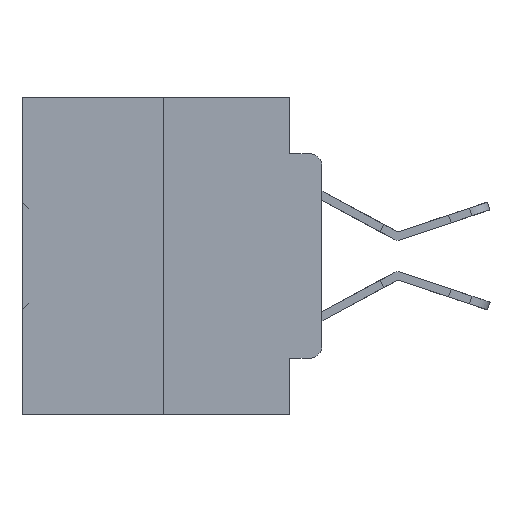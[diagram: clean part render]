
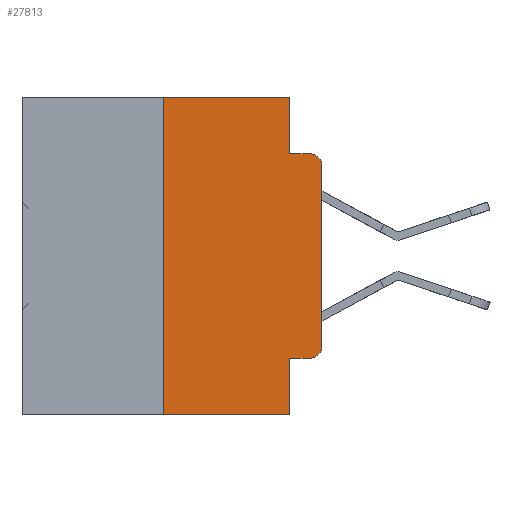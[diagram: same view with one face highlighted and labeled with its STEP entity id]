
A CAD part, left-side view. The second image highlights one B-rep face of the part: STEP entity #27813.
In plain terms, the highlighted planar face has unit normal (-1, 0, 0).
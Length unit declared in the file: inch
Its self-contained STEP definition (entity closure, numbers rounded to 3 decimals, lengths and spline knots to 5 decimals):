
#377 = CARTESIAN_POINT ( 'NONE',  ( 0., 0.02, -0.1085 ) ) ;
#458 = ORIENTED_EDGE ( 'NONE', *, *, #30787, .F. ) ;
#922 = EDGE_CURVE ( 'NONE', #39121, #20707, #31817, .T. ) ;
#1059 = ORIENTED_EDGE ( 'NONE', *, *, #10953, .T. ) ;
#1646 = AXIS2_PLACEMENT_3D ( 'NONE', #377, #25397, #3237 ) ;
#1842 = ORIENTED_EDGE ( 'NONE', *, *, #34282, .T. ) ;
#2222 = CARTESIAN_POINT ( 'NONE',  ( 0., 0.051, -0.4115 ) ) ;
#3047 = DIRECTION ( 'NONE',  ( 0., 0., -1. ) ) ;
#3237 = DIRECTION ( 'NONE',  ( 0., 0., -1. ) ) ;
#3352 = LINE ( 'NONE', #37410, #21330 ) ;
#3998 = ORIENTED_EDGE ( 'NONE', *, *, #922, .F. ) ;
#4607 = CARTESIAN_POINT ( 'NONE',  ( 0., 0.051, 0. ) ) ;
#4896 = VERTEX_POINT ( 'NONE', #10199 ) ;
#5140 = EDGE_CURVE ( 'NONE', #37113, #7721, #8567, .T. ) ;
#5470 = FACE_OUTER_BOUND ( 'NONE', #26288, .T. ) ;
#5707 = ORIENTED_EDGE ( 'NONE', *, *, #20006, .T. ) ;
#6182 = CARTESIAN_POINT ( 'NONE',  ( 0., 0.25, 0. ) ) ;
#6184 = ORIENTED_EDGE ( 'NONE', *, *, #12628, .F. ) ;
#6876 = CARTESIAN_POINT ( 'NONE',  ( 0., 0.051, -0.0885 ) ) ;
#7721 = VERTEX_POINT ( 'NONE', #10464 ) ;
#8567 = LINE ( 'NONE', #32364, #11851 ) ;
#8729 = CIRCLE ( 'NONE', #1646, 0.02 ) ;
#9619 = VERTEX_POINT ( 'NONE', #39249 ) ;
#10199 = CARTESIAN_POINT ( 'NONE',  ( 0., 0., -0.3915 ) ) ;
#10464 = CARTESIAN_POINT ( 'NONE',  ( 0., 0.02, -0.0885 ) ) ;
#10778 = CIRCLE ( 'NONE', #11408, 0.02 ) ;
#10953 = EDGE_CURVE ( 'NONE', #39121, #31346, #32854, .T. ) ;
#11408 = AXIS2_PLACEMENT_3D ( 'NONE', #16907, #32036, #20530 ) ;
#11587 = DIRECTION ( 'NONE',  ( 0., -1., 0. ) ) ;
#11851 = VECTOR ( 'NONE', #11587, 39.37008 ) ;
#12628 = EDGE_CURVE ( 'NONE', #38795, #37113, #25783, .T. ) ;
#13248 = DIRECTION ( 'NONE',  ( 0., 0., 1. ) ) ;
#13887 = CARTESIAN_POINT ( 'NONE',  ( 0., 0.051, 0. ) ) ;
#14482 = EDGE_CURVE ( 'NONE', #37508, #20707, #3352, .T. ) ;
#15506 = CARTESIAN_POINT ( 'NONE',  ( 0., 0.25, 0. ) ) ;
#16087 = DIRECTION ( 'NONE',  ( 0., 0., -1. ) ) ;
#16580 = ORIENTED_EDGE ( 'NONE', *, *, #14482, .T. ) ;
#16879 = ORIENTED_EDGE ( 'NONE', *, *, #5140, .F. ) ;
#16907 = CARTESIAN_POINT ( 'NONE',  ( 0., 0.02, -0.3915 ) ) ;
#17319 = CARTESIAN_POINT ( 'NONE',  ( 0., 0.473, 0. ) ) ;
#17368 = ORIENTED_EDGE ( 'NONE', *, *, #39757, .T. ) ;
#18345 = PLANE ( 'NONE',  #19386 ) ;
#18455 = DIRECTION ( 'NONE',  ( 0., 0., 1. ) ) ;
#18849 = DIRECTION ( 'NONE',  ( 0., -1., 0. ) ) ;
#19386 = AXIS2_PLACEMENT_3D ( 'NONE', #36103, #30049, #3047 ) ;
#20006 = EDGE_CURVE ( 'NONE', #9619, #7721, #8729, .T. ) ;
#20530 = DIRECTION ( 'NONE',  ( 0., 0., -1. ) ) ;
#20707 = VERTEX_POINT ( 'NONE', #31081 ) ;
#20748 = CARTESIAN_POINT ( 'NONE',  ( 0., 0.25, -0.5 ) ) ;
#20751 = DIRECTION ( 'NONE',  ( 0., -1., 0. ) ) ;
#20870 = VECTOR ( 'NONE', #20751, 39.37008 ) ;
#21330 = VECTOR ( 'NONE', #18849, 39.37008 ) ;
#23921 = VERTEX_POINT ( 'NONE', #15506 ) ;
#24989 = VECTOR ( 'NONE', #13248, 39.37008 ) ;
#25122 = VECTOR ( 'NONE', #35687, 39.37008 ) ;
#25397 = DIRECTION ( 'NONE',  ( -1., 0., 0. ) ) ;
#25742 = CARTESIAN_POINT ( 'NONE',  ( 0., 0., 0. ) ) ;
#25783 = LINE ( 'NONE', #13887, #26413 ) ;
#26288 = EDGE_LOOP ( 'NONE', ( #17368, #5707, #16879, #6184, #458, #37160, #16580, #3998, #1059, #1842 ) ) ;
#26413 = VECTOR ( 'NONE', #35250, 39.37008 ) ;
#27813 = ADVANCED_FACE ( 'NONE', ( #5470 ), #18345, .F. ) ;
#27913 = VECTOR ( 'NONE', #18455, 39.37008 ) ;
#28613 = CARTESIAN_POINT ( 'NONE',  ( 0., 0.051, -0.4115 ) ) ;
#30049 = DIRECTION ( 'NONE',  ( 1., 0., 0. ) ) ;
#30787 = EDGE_CURVE ( 'NONE', #23921, #38795, #36282, .T. ) ;
#31081 = CARTESIAN_POINT ( 'NONE',  ( 0., 0.051, -0.5 ) ) ;
#31346 = VERTEX_POINT ( 'NONE', #32608 ) ;
#31533 = EDGE_CURVE ( 'NONE', #37508, #23921, #33796, .T. ) ;
#31817 = LINE ( 'NONE', #4607, #33098 ) ;
#31980 = LINE ( 'NONE', #25742, #24989 ) ;
#32036 = DIRECTION ( 'NONE',  ( -1., 0., 0. ) ) ;
#32364 = CARTESIAN_POINT ( 'NONE',  ( 0., 0.051, -0.0885 ) ) ;
#32608 = CARTESIAN_POINT ( 'NONE',  ( 0., 0.02, -0.4115 ) ) ;
#32854 = LINE ( 'NONE', #2222, #25122 ) ;
#33098 = VECTOR ( 'NONE', #16087, 39.37008 ) ;
#33796 = LINE ( 'NONE', #6182, #27913 ) ;
#34282 = EDGE_CURVE ( 'NONE', #31346, #4896, #10778, .T. ) ;
#35250 = DIRECTION ( 'NONE',  ( 0., 0., -1. ) ) ;
#35687 = DIRECTION ( 'NONE',  ( 0., -1., 0. ) ) ;
#36103 = CARTESIAN_POINT ( 'NONE',  ( 0., 0.473, 0. ) ) ;
#36282 = LINE ( 'NONE', #17319, #20870 ) ;
#37113 = VERTEX_POINT ( 'NONE', #6876 ) ;
#37160 = ORIENTED_EDGE ( 'NONE', *, *, #31533, .F. ) ;
#37410 = CARTESIAN_POINT ( 'NONE',  ( 0., 0.473, -0.5 ) ) ;
#37508 = VERTEX_POINT ( 'NONE', #20748 ) ;
#38514 = CARTESIAN_POINT ( 'NONE',  ( 0., 0.051, 0. ) ) ;
#38795 = VERTEX_POINT ( 'NONE', #38514 ) ;
#39121 = VERTEX_POINT ( 'NONE', #28613 ) ;
#39249 = CARTESIAN_POINT ( 'NONE',  ( 0., 0., -0.1085 ) ) ;
#39757 = EDGE_CURVE ( 'NONE', #4896, #9619, #31980, .T. ) ;
